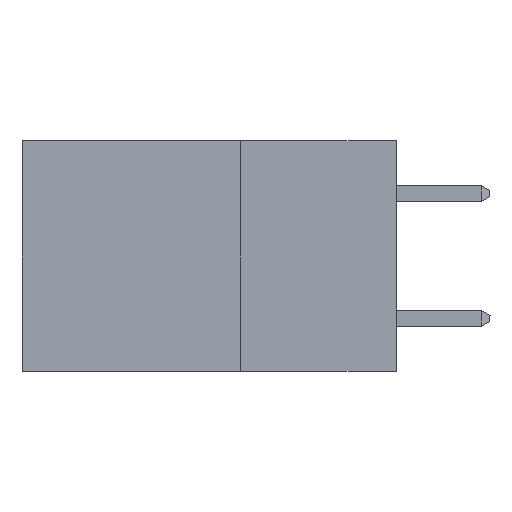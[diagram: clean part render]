
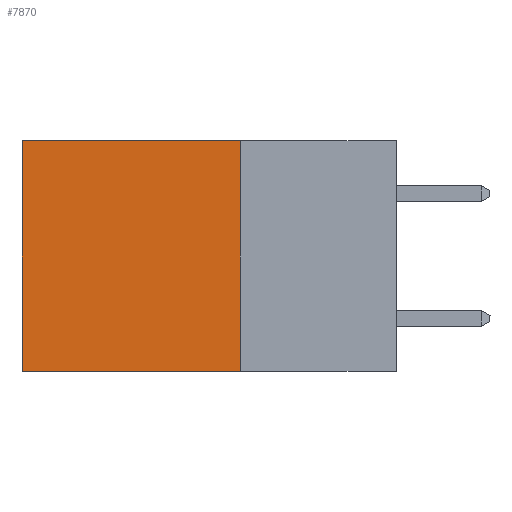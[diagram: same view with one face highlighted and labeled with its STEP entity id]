
A CAD part, left-side view. The second image highlights one B-rep face of the part: STEP entity #7870.
In plain terms, the highlighted planar face has unit normal (-1, 0, 0).
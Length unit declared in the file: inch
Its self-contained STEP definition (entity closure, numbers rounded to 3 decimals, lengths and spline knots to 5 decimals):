
#104 = VECTOR ( 'NONE', #3023, 39.37008 ) ;
#744 = EDGE_CURVE ( 'NONE', #2838, #1197, #7006, .T. ) ;
#799 = DIRECTION ( 'NONE',  ( 0., 1., 0. ) ) ;
#815 = EDGE_CURVE ( 'NONE', #2565, #2838, #3529, .T. ) ;
#1098 = DIRECTION ( 'NONE',  ( 0., 0., -1. ) ) ;
#1117 = LINE ( 'NONE', #5398, #4529 ) ;
#1197 = VERTEX_POINT ( 'NONE', #4971 ) ;
#1509 = VECTOR ( 'NONE', #799, 39.37008 ) ;
#2198 = CARTESIAN_POINT ( 'NONE',  ( 0.2615, 0.25, -0.37 ) ) ;
#2565 = VERTEX_POINT ( 'NONE', #5055 ) ;
#2838 = VERTEX_POINT ( 'NONE', #4945 ) ;
#2867 = DIRECTION ( 'NONE',  ( 0., 0., -1. ) ) ;
#2986 = VERTEX_POINT ( 'NONE', #3829 ) ;
#3023 = DIRECTION ( 'NONE',  ( 0., 0., -1. ) ) ;
#3138 = ORIENTED_EDGE ( 'NONE', *, *, #815, .T. ) ;
#3180 = CARTESIAN_POINT ( 'NONE',  ( 0.2615, 0.25, -0.37 ) ) ;
#3529 = LINE ( 'NONE', #6591, #1509 ) ;
#3829 = CARTESIAN_POINT ( 'NONE',  ( 0.2615, 0.25, -0.37 ) ) ;
#3888 = AXIS2_PLACEMENT_3D ( 'NONE', #2198, #6773, #2867 ) ;
#4005 = EDGE_CURVE ( 'NONE', #2986, #1197, #1117, .T. ) ;
#4323 = ORIENTED_EDGE ( 'NONE', *, *, #7514, .F. ) ;
#4529 = VECTOR ( 'NONE', #5371, 39.37008 ) ;
#4868 = CARTESIAN_POINT ( 'NONE',  ( 0.2615, 0.6, -0.37 ) ) ;
#4945 = CARTESIAN_POINT ( 'NONE',  ( 0.2615, 0.6, 0. ) ) ;
#4971 = CARTESIAN_POINT ( 'NONE',  ( 0.2615, 0.6, -0.37 ) ) ;
#5055 = CARTESIAN_POINT ( 'NONE',  ( 0.2615, 0.25, 0. ) ) ;
#5371 = DIRECTION ( 'NONE',  ( 0., 1., 0. ) ) ;
#5398 = CARTESIAN_POINT ( 'NONE',  ( 0.2615, 0.25, -0.37 ) ) ;
#5436 = FACE_OUTER_BOUND ( 'NONE', #5760, .T. ) ;
#5760 = EDGE_LOOP ( 'NONE', ( #6843, #5857, #4323, #3138 ) ) ;
#5857 = ORIENTED_EDGE ( 'NONE', *, *, #4005, .F. ) ;
#6144 = PLANE ( 'NONE',  #3888 ) ;
#6342 = LINE ( 'NONE', #3180, #7850 ) ;
#6591 = CARTESIAN_POINT ( 'NONE',  ( 0.2615, 0.25, 0. ) ) ;
#6773 = DIRECTION ( 'NONE',  ( 1., 0., 0. ) ) ;
#6843 = ORIENTED_EDGE ( 'NONE', *, *, #744, .T. ) ;
#7006 = LINE ( 'NONE', #4868, #104 ) ;
#7514 = EDGE_CURVE ( 'NONE', #2565, #2986, #6342, .T. ) ;
#7850 = VECTOR ( 'NONE', #1098, 39.37008 ) ;
#7870 = ADVANCED_FACE ( 'NONE', ( #5436 ), #6144, .F. ) ;
